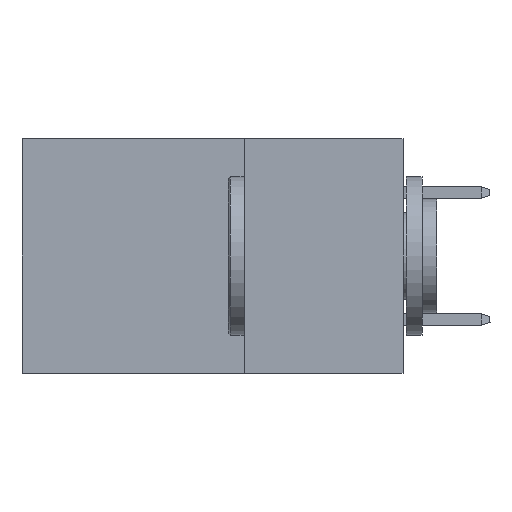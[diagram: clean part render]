
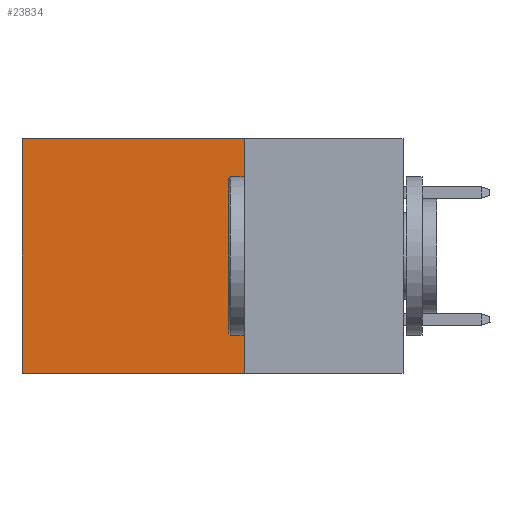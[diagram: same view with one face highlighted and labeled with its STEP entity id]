
A CAD part, left-side view. The second image highlights one B-rep face of the part: STEP entity #23834.
In plain terms, the highlighted planar face has unit normal (-1, 0, 0).
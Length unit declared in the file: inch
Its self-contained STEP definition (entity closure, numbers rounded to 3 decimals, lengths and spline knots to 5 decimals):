
#73 = EDGE_CURVE ( 'NONE', #12713, #16694, #18288, .T. ) ;
#1768 = LINE ( 'NONE', #4819, #39899 ) ;
#2613 = VECTOR ( 'NONE', #4192, 39.37008 ) ;
#2839 = CARTESIAN_POINT ( 'NONE',  ( 0.2875, 0.25, 0. ) ) ;
#4192 = DIRECTION ( 'NONE',  ( 0., 1., 0. ) ) ;
#4355 = EDGE_CURVE ( 'NONE', #16694, #15799, #1768, .T. ) ;
#4819 = CARTESIAN_POINT ( 'NONE',  ( 0.2875, 0.6, 0. ) ) ;
#5986 = PLANE ( 'NONE',  #20402 ) ;
#7823 = ORIENTED_EDGE ( 'NONE', *, *, #11922, .F. ) ;
#9431 = DIRECTION ( 'NONE',  ( 1., 0., 0. ) ) ;
#9573 = DIRECTION ( 'NONE',  ( 0., 0., -1. ) ) ;
#10190 = ORIENTED_EDGE ( 'NONE', *, *, #73, .T. ) ;
#10332 = VERTEX_POINT ( 'NONE', #34190 ) ;
#10627 = EDGE_LOOP ( 'NONE', ( #11648, #11858, #7823, #10190 ) ) ;
#11350 = DIRECTION ( 'NONE',  ( 0., 0., -1. ) ) ;
#11648 = ORIENTED_EDGE ( 'NONE', *, *, #4355, .T. ) ;
#11858 = ORIENTED_EDGE ( 'NONE', *, *, #35788, .F. ) ;
#11899 = FACE_OUTER_BOUND ( 'NONE', #10627, .T. ) ;
#11922 = EDGE_CURVE ( 'NONE', #12713, #10332, #27689, .T. ) ;
#12713 = VERTEX_POINT ( 'NONE', #26372 ) ;
#15799 = VERTEX_POINT ( 'NONE', #15929 ) ;
#15929 = CARTESIAN_POINT ( 'NONE',  ( 0.2875, 0.6, -0.37 ) ) ;
#16694 = VERTEX_POINT ( 'NONE', #34436 ) ;
#16906 = VECTOR ( 'NONE', #9573, 39.37008 ) ;
#18288 = LINE ( 'NONE', #24164, #19881 ) ;
#19852 = LINE ( 'NONE', #29411, #2613 ) ;
#19881 = VECTOR ( 'NONE', #36592, 39.37008 ) ;
#20402 = AXIS2_PLACEMENT_3D ( 'NONE', #33614, #9431, #24061 ) ;
#23834 = ADVANCED_FACE ( 'NONE', ( #11899 ), #5986, .F. ) ;
#24061 = DIRECTION ( 'NONE',  ( 0., 0., -1. ) ) ;
#24164 = CARTESIAN_POINT ( 'NONE',  ( 0.2875, 0.25, 0. ) ) ;
#26372 = CARTESIAN_POINT ( 'NONE',  ( 0.2875, 0.25, 0. ) ) ;
#27689 = LINE ( 'NONE', #2839, #16906 ) ;
#29411 = CARTESIAN_POINT ( 'NONE',  ( 0.2875, 0.25, -0.37 ) ) ;
#33614 = CARTESIAN_POINT ( 'NONE',  ( 0.2875, 0.25, 0. ) ) ;
#34190 = CARTESIAN_POINT ( 'NONE',  ( 0.2875, 0.25, -0.37 ) ) ;
#34436 = CARTESIAN_POINT ( 'NONE',  ( 0.2875, 0.6, 0. ) ) ;
#35788 = EDGE_CURVE ( 'NONE', #10332, #15799, #19852, .T. ) ;
#36592 = DIRECTION ( 'NONE',  ( 0., 1., 0. ) ) ;
#39899 = VECTOR ( 'NONE', #11350, 39.37008 ) ;
